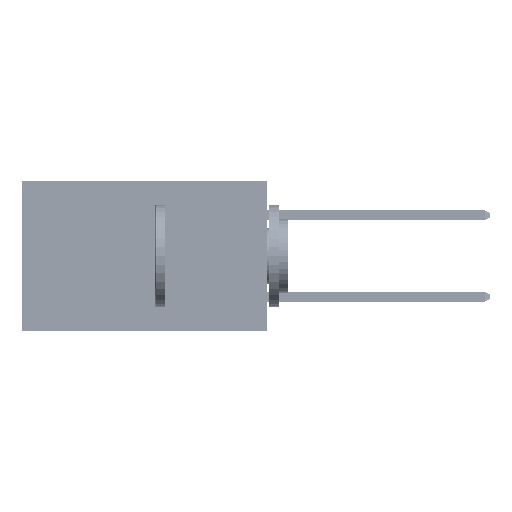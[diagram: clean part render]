
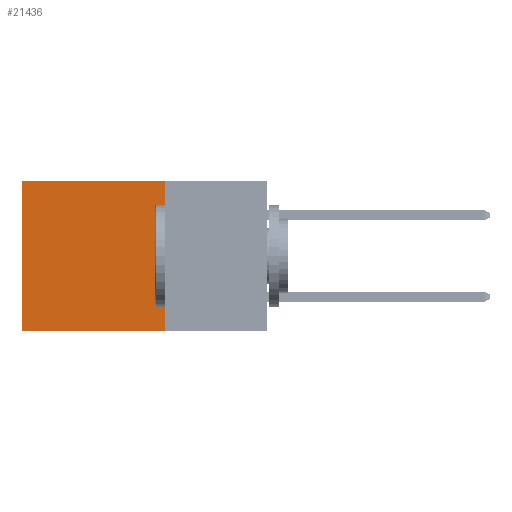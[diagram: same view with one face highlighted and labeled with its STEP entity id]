
A CAD part, left-side view. The second image highlights one B-rep face of the part: STEP entity #21436.
In plain terms, the highlighted planar face has unit normal (-1, 0, 0).
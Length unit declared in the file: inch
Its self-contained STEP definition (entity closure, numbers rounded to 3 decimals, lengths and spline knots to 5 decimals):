
#1994 = LINE ( 'NONE', #34220, #34492 ) ;
#2145 = CARTESIAN_POINT ( 'NONE',  ( 0.2875, 0.6, -0.37 ) ) ;
#2388 = VERTEX_POINT ( 'NONE', #16349 ) ;
#4047 = DIRECTION ( 'NONE',  ( 0., 0., -1. ) ) ;
#6413 = DIRECTION ( 'NONE',  ( 1., 0., 0. ) ) ;
#7486 = VERTEX_POINT ( 'NONE', #13677 ) ;
#7487 = DIRECTION ( 'NONE',  ( 0., 1., 0. ) ) ;
#9031 = VECTOR ( 'NONE', #22303, 39.37008 ) ;
#12426 = ORIENTED_EDGE ( 'NONE', *, *, #40995, .T. ) ;
#13677 = CARTESIAN_POINT ( 'NONE',  ( 0.2875, 0.25, -0.37 ) ) ;
#14302 = CARTESIAN_POINT ( 'NONE',  ( 0.2875, 0.25, 0. ) ) ;
#14401 = CARTESIAN_POINT ( 'NONE',  ( 0.2875, 0.25, 0. ) ) ;
#16295 = ORIENTED_EDGE ( 'NONE', *, *, #30757, .F. ) ;
#16349 = CARTESIAN_POINT ( 'NONE',  ( 0.2875, 0.6, 0. ) ) ;
#19319 = CARTESIAN_POINT ( 'NONE',  ( 0.2875, 0.6, 0. ) ) ;
#20201 = VERTEX_POINT ( 'NONE', #30228 ) ;
#20203 = VECTOR ( 'NONE', #4047, 39.37008 ) ;
#21399 = AXIS2_PLACEMENT_3D ( 'NONE', #14302, #6413, #25933 ) ;
#21436 = ADVANCED_FACE ( 'NONE', ( #43622 ), #49044, .F. ) ;
#21655 = VERTEX_POINT ( 'NONE', #2145 ) ;
#22303 = DIRECTION ( 'NONE',  ( 0., 0., -1. ) ) ;
#22757 = DIRECTION ( 'NONE',  ( 0., 1., 0. ) ) ;
#25713 = LINE ( 'NONE', #19319, #20203 ) ;
#25933 = DIRECTION ( 'NONE',  ( 0., 0., -1. ) ) ;
#27575 = EDGE_CURVE ( 'NONE', #7486, #21655, #39570, .T. ) ;
#29886 = VECTOR ( 'NONE', #7487, 39.37008 ) ;
#30228 = CARTESIAN_POINT ( 'NONE',  ( 0.2875, 0.25, 0. ) ) ;
#30757 = EDGE_CURVE ( 'NONE', #20201, #7486, #40418, .T. ) ;
#34220 = CARTESIAN_POINT ( 'NONE',  ( 0.2875, 0.25, 0. ) ) ;
#34492 = VECTOR ( 'NONE', #22757, 39.37008 ) ;
#38379 = ORIENTED_EDGE ( 'NONE', *, *, #45807, .T. ) ;
#39570 = LINE ( 'NONE', #45435, #29886 ) ;
#40418 = LINE ( 'NONE', #14401, #9031 ) ;
#40995 = EDGE_CURVE ( 'NONE', #20201, #2388, #1994, .T. ) ;
#43622 = FACE_OUTER_BOUND ( 'NONE', #46473, .T. ) ;
#45009 = ORIENTED_EDGE ( 'NONE', *, *, #27575, .F. ) ;
#45435 = CARTESIAN_POINT ( 'NONE',  ( 0.2875, 0.25, -0.37 ) ) ;
#45807 = EDGE_CURVE ( 'NONE', #2388, #21655, #25713, .T. ) ;
#46473 = EDGE_LOOP ( 'NONE', ( #38379, #45009, #16295, #12426 ) ) ;
#49044 = PLANE ( 'NONE',  #21399 ) ;
